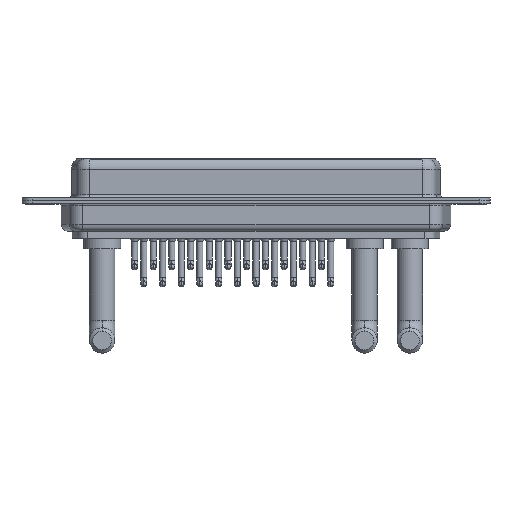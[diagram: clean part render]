
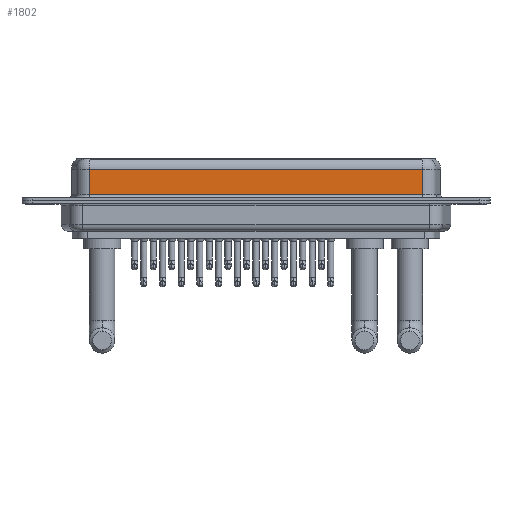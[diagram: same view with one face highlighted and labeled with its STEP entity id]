
A CAD part, front view. The second image highlights one B-rep face of the part: STEP entity #1802.
In plain terms, the highlighted planar face has unit normal (0, -1, 0).
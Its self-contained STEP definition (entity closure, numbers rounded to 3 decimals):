
#72 = LINE ( 'NONE', #4994, #14737 ) ;
#352 = VECTOR ( 'NONE', #10514, 1000. ) ;
#1176 = PLANE ( 'NONE',  #6958 ) ;
#1333 = CARTESIAN_POINT ( 'NONE',  ( 7.038, -3.95, 6.4 ) ) ;
#1360 = VERTEX_POINT ( 'NONE', #11225 ) ;
#1802 = ADVANCED_FACE ( 'NONE', ( #14992 ), #1176, .F. ) ;
#1978 = VERTEX_POINT ( 'NONE', #8746 ) ;
#2222 = VECTOR ( 'NONE', #16118, 1000. ) ;
#2454 = LINE ( 'NONE', #19575, #2222 ) ;
#3162 = EDGE_CURVE ( 'NONE', #4236, #1978, #16881, .T. ) ;
#4236 = VERTEX_POINT ( 'NONE', #20616 ) ;
#4798 = EDGE_CURVE ( 'NONE', #1360, #1978, #2454, .T. ) ;
#4994 = CARTESIAN_POINT ( 'NONE',  ( 56.462, -3.95, 4.65 ) ) ;
#5814 = ORIENTED_EDGE ( 'NONE', *, *, #6435, .T. ) ;
#6435 = EDGE_CURVE ( 'NONE', #1360, #15879, #72, .T. ) ;
#6958 = AXIS2_PLACEMENT_3D ( 'NONE', #7868, #21333, #21776 ) ;
#7868 = CARTESIAN_POINT ( 'NONE',  ( 56.462, -3.95, 6.4 ) ) ;
#8746 = CARTESIAN_POINT ( 'NONE',  ( 56.462, -3.95, 0.9 ) ) ;
#8769 = DIRECTION ( 'NONE',  ( -1., 0., 0. ) ) ;
#9848 = ORIENTED_EDGE ( 'NONE', *, *, #4798, .F. ) ;
#10226 = DIRECTION ( 'NONE',  ( 0., 0., -1. ) ) ;
#10514 = DIRECTION ( 'NONE',  ( 1., 0., 0. ) ) ;
#11225 = CARTESIAN_POINT ( 'NONE',  ( 56.462, -3.95, 4.65 ) ) ;
#12378 = VECTOR ( 'NONE', #10226, 1000. ) ;
#14737 = VECTOR ( 'NONE', #8769, 1000. ) ;
#14992 = FACE_OUTER_BOUND ( 'NONE', #18978, .T. ) ;
#15837 = CARTESIAN_POINT ( 'NONE',  ( 7.038, -3.95, 4.65 ) ) ;
#15879 = VERTEX_POINT ( 'NONE', #15837 ) ;
#16118 = DIRECTION ( 'NONE',  ( 0., 0., -1. ) ) ;
#16881 = LINE ( 'NONE', #20556, #352 ) ;
#18978 = EDGE_LOOP ( 'NONE', ( #9848, #5814, #21549, #19033 ) ) ;
#19033 = ORIENTED_EDGE ( 'NONE', *, *, #3162, .T. ) ;
#19575 = CARTESIAN_POINT ( 'NONE',  ( 56.462, -3.95, 6.4 ) ) ;
#20510 = EDGE_CURVE ( 'NONE', #15879, #4236, #21815, .T. ) ;
#20556 = CARTESIAN_POINT ( 'NONE',  ( 56.462, -3.95, 0.9 ) ) ;
#20616 = CARTESIAN_POINT ( 'NONE',  ( 7.038, -3.95, 0.9 ) ) ;
#21333 = DIRECTION ( 'NONE',  ( 0., 1., 0. ) ) ;
#21549 = ORIENTED_EDGE ( 'NONE', *, *, #20510, .T. ) ;
#21776 = DIRECTION ( 'NONE',  ( 0., 0., 1. ) ) ;
#21815 = LINE ( 'NONE', #1333, #12378 ) ;
